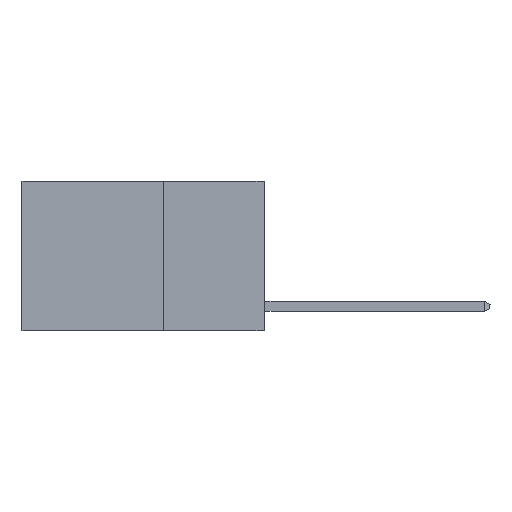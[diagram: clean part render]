
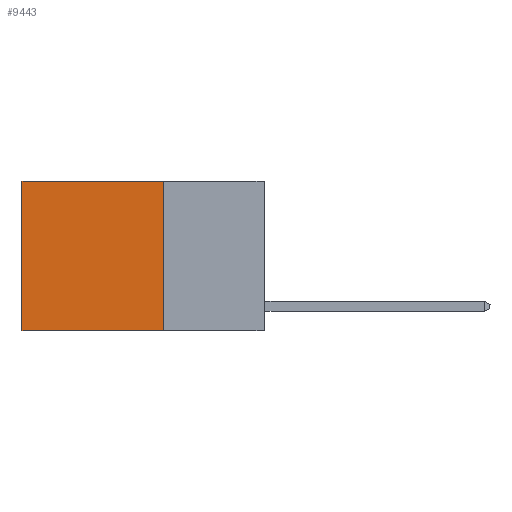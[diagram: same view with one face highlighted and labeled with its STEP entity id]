
A CAD part, left-side view. The second image highlights one B-rep face of the part: STEP entity #9443.
In plain terms, the highlighted planar face has unit normal (-1, 0, 0).
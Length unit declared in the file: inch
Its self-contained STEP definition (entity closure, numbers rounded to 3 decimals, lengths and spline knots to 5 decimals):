
#1291 = DIRECTION ( 'NONE',  ( 0., 0., -1. ) ) ;
#1610 = ORIENTED_EDGE ( 'NONE', *, *, #9244, .T. ) ;
#2565 = PLANE ( 'NONE',  #7584 ) ;
#2659 = VECTOR ( 'NONE', #10809, 39.37008 ) ;
#3105 = VERTEX_POINT ( 'NONE', #11265 ) ;
#3380 = CARTESIAN_POINT ( 'NONE',  ( 0.2625, 0.25, -0.37 ) ) ;
#4780 = VERTEX_POINT ( 'NONE', #3380 ) ;
#5679 = CARTESIAN_POINT ( 'NONE',  ( 0.2625, 0.6, 0. ) ) ;
#5894 = CARTESIAN_POINT ( 'NONE',  ( 0.2625, 0.25, 0. ) ) ;
#5895 = LINE ( 'NONE', #15137, #8664 ) ;
#6143 = VERTEX_POINT ( 'NONE', #7230 ) ;
#6190 = VERTEX_POINT ( 'NONE', #6404 ) ;
#6294 = EDGE_CURVE ( 'NONE', #4780, #6190, #14359, .T. ) ;
#6404 = CARTESIAN_POINT ( 'NONE',  ( 0.2625, 0.6, -0.37 ) ) ;
#7230 = CARTESIAN_POINT ( 'NONE',  ( 0.2625, 0.6, 0. ) ) ;
#7378 = CARTESIAN_POINT ( 'NONE',  ( 0.2625, 0.25, -0.37 ) ) ;
#7535 = CARTESIAN_POINT ( 'NONE',  ( 0.2625, 0.25, 0. ) ) ;
#7584 = AXIS2_PLACEMENT_3D ( 'NONE', #5894, #8275, #1291 ) ;
#8203 = EDGE_CURVE ( 'NONE', #3105, #4780, #5895, .T. ) ;
#8270 = LINE ( 'NONE', #7535, #9900 ) ;
#8275 = DIRECTION ( 'NONE',  ( 1., 0., 0. ) ) ;
#8664 = VECTOR ( 'NONE', #15024, 39.37008 ) ;
#9131 = ORIENTED_EDGE ( 'NONE', *, *, #8203, .F. ) ;
#9244 = EDGE_CURVE ( 'NONE', #3105, #6143, #8270, .T. ) ;
#9361 = DIRECTION ( 'NONE',  ( 0., 0., -1. ) ) ;
#9443 = ADVANCED_FACE ( 'NONE', ( #14455 ), #2565, .F. ) ;
#9900 = VECTOR ( 'NONE', #12114, 39.37008 ) ;
#10183 = EDGE_CURVE ( 'NONE', #6143, #6190, #11885, .T. ) ;
#10809 = DIRECTION ( 'NONE',  ( 0., 1., 0. ) ) ;
#11265 = CARTESIAN_POINT ( 'NONE',  ( 0.2625, 0.25, 0. ) ) ;
#11885 = LINE ( 'NONE', #5679, #13504 ) ;
#12114 = DIRECTION ( 'NONE',  ( 0., 1., 0. ) ) ;
#13333 = ORIENTED_EDGE ( 'NONE', *, *, #6294, .F. ) ;
#13504 = VECTOR ( 'NONE', #9361, 39.37008 ) ;
#13597 = ORIENTED_EDGE ( 'NONE', *, *, #10183, .T. ) ;
#13661 = EDGE_LOOP ( 'NONE', ( #13597, #13333, #9131, #1610 ) ) ;
#14359 = LINE ( 'NONE', #7378, #2659 ) ;
#14455 = FACE_OUTER_BOUND ( 'NONE', #13661, .T. ) ;
#15024 = DIRECTION ( 'NONE',  ( 0., 0., -1. ) ) ;
#15137 = CARTESIAN_POINT ( 'NONE',  ( 0.2625, 0.25, 0. ) ) ;
